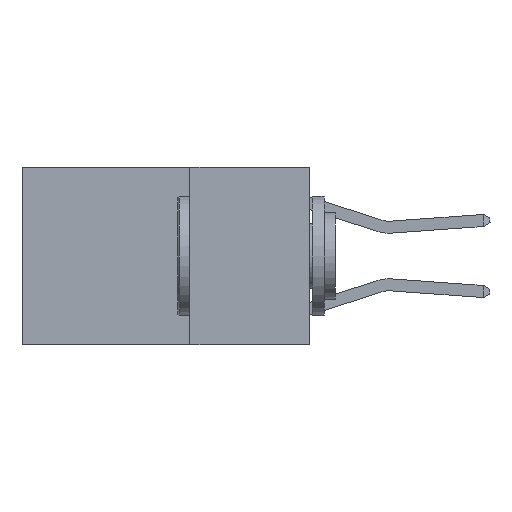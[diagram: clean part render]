
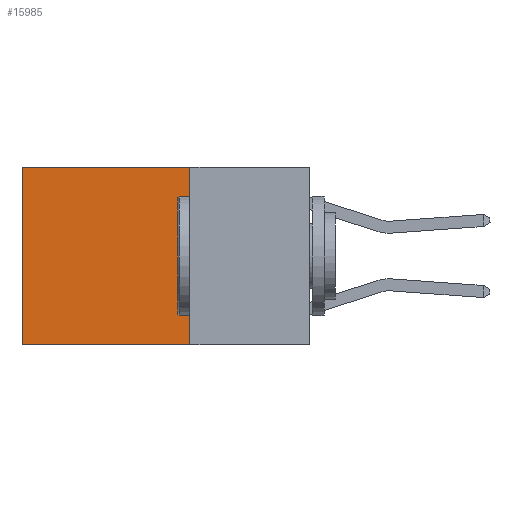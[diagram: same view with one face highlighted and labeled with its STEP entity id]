
A CAD part, left-side view. The second image highlights one B-rep face of the part: STEP entity #15985.
In plain terms, the highlighted planar face has unit normal (-1, 0, 0).
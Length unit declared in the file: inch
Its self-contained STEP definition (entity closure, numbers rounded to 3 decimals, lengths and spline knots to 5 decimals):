
#1111 = EDGE_CURVE ( 'NONE', #15977, #15675, #19245, .T. ) ;
#1504 = LINE ( 'NONE', #12200, #2635 ) ;
#1737 = CARTESIAN_POINT ( 'NONE',  ( 0.2625, 0.6, -0.37 ) ) ;
#2635 = VECTOR ( 'NONE', #9949, 39.37008 ) ;
#3890 = ORIENTED_EDGE ( 'NONE', *, *, #1111, .T. ) ;
#4759 = EDGE_CURVE ( 'NONE', #10978, #15977, #1504, .T. ) ;
#5825 = VECTOR ( 'NONE', #13011, 39.37008 ) ;
#6717 = DIRECTION ( 'NONE',  ( 0., 0., -1. ) ) ;
#6832 = CARTESIAN_POINT ( 'NONE',  ( 0.2625, 0.25, 0. ) ) ;
#7450 = CARTESIAN_POINT ( 'NONE',  ( 0.2625, 0.25, 0. ) ) ;
#7923 = VECTOR ( 'NONE', #6717, 39.37008 ) ;
#9067 = CARTESIAN_POINT ( 'NONE',  ( 0.2625, 0.25, 0. ) ) ;
#9949 = DIRECTION ( 'NONE',  ( 0., 1., 0. ) ) ;
#10978 = VERTEX_POINT ( 'NONE', #7450 ) ;
#12200 = CARTESIAN_POINT ( 'NONE',  ( 0.2625, 0.25, 0. ) ) ;
#12375 = DIRECTION ( 'NONE',  ( 0., 1., 0. ) ) ;
#12826 = ORIENTED_EDGE ( 'NONE', *, *, #4759, .T. ) ;
#13011 = DIRECTION ( 'NONE',  ( 0., 0., -1. ) ) ;
#13090 = ORIENTED_EDGE ( 'NONE', *, *, #14700, .F. ) ;
#14402 = CARTESIAN_POINT ( 'NONE',  ( 0.2625, 0.25, -0.37 ) ) ;
#14700 = EDGE_CURVE ( 'NONE', #10978, #18104, #23653, .T. ) ;
#15233 = PLANE ( 'NONE',  #26426 ) ;
#15369 = DIRECTION ( 'NONE',  ( 0., 0., -1. ) ) ;
#15675 = VERTEX_POINT ( 'NONE', #1737 ) ;
#15977 = VERTEX_POINT ( 'NONE', #25476 ) ;
#15985 = ADVANCED_FACE ( 'NONE', ( #19689 ), #15233, .F. ) ;
#17262 = DIRECTION ( 'NONE',  ( 1., 0., 0. ) ) ;
#18104 = VERTEX_POINT ( 'NONE', #25812 ) ;
#18481 = VECTOR ( 'NONE', #12375, 39.37008 ) ;
#18729 = LINE ( 'NONE', #14402, #18481 ) ;
#19245 = LINE ( 'NONE', #21263, #7923 ) ;
#19341 = ORIENTED_EDGE ( 'NONE', *, *, #23018, .F. ) ;
#19689 = FACE_OUTER_BOUND ( 'NONE', #25691, .T. ) ;
#21263 = CARTESIAN_POINT ( 'NONE',  ( 0.2625, 0.6, 0. ) ) ;
#23018 = EDGE_CURVE ( 'NONE', #18104, #15675, #18729, .T. ) ;
#23653 = LINE ( 'NONE', #6832, #5825 ) ;
#25476 = CARTESIAN_POINT ( 'NONE',  ( 0.2625, 0.6, 0. ) ) ;
#25691 = EDGE_LOOP ( 'NONE', ( #3890, #19341, #13090, #12826 ) ) ;
#25812 = CARTESIAN_POINT ( 'NONE',  ( 0.2625, 0.25, -0.37 ) ) ;
#26426 = AXIS2_PLACEMENT_3D ( 'NONE', #9067, #17262, #15369 ) ;
